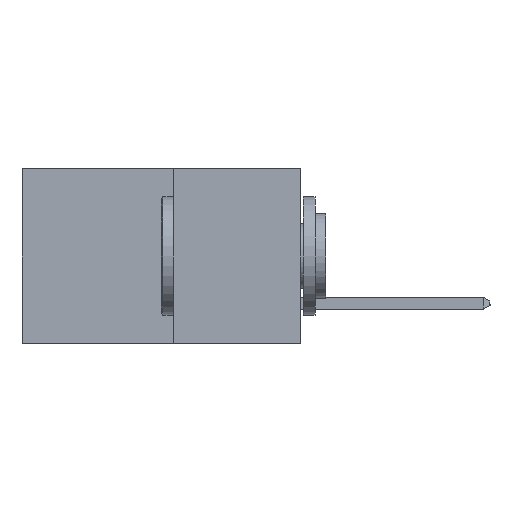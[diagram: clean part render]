
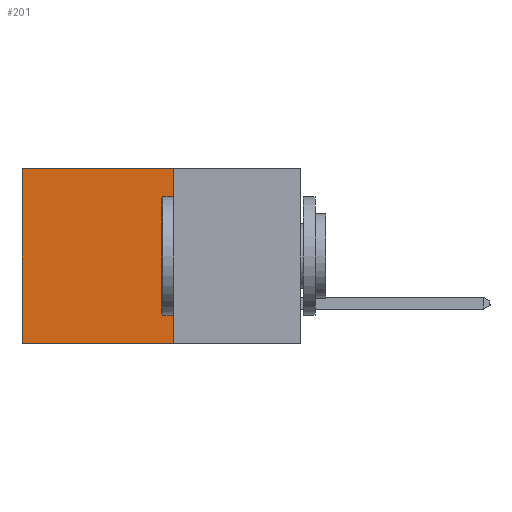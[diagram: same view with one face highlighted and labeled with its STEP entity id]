
A CAD part, left-side view. The second image highlights one B-rep face of the part: STEP entity #201.
In plain terms, the highlighted planar face has unit normal (-1, 0, 0).
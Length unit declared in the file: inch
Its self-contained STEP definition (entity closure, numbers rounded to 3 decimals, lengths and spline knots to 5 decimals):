
#201 = ADVANCED_FACE ( 'NONE', ( #12856 ), #9001, .F. ) ;
#291 = DIRECTION ( 'NONE',  ( 0., 1., 0. ) ) ;
#618 = ORIENTED_EDGE ( 'NONE', *, *, #7267, .T. ) ;
#1165 = ORIENTED_EDGE ( 'NONE', *, *, #3580, .F. ) ;
#1316 = LINE ( 'NONE', #10894, #13459 ) ;
#1512 = ORIENTED_EDGE ( 'NONE', *, *, #8063, .F. ) ;
#1718 = DIRECTION ( 'NONE',  ( 0., 0., -1. ) ) ;
#1719 = DIRECTION ( 'NONE',  ( 1., 0., 0. ) ) ;
#1788 = ORIENTED_EDGE ( 'NONE', *, *, #15020, .T. ) ;
#2161 = CARTESIAN_POINT ( 'NONE',  ( 0.277, 0.27, -0.37 ) ) ;
#2297 = CARTESIAN_POINT ( 'NONE',  ( 0.277, 0.59, 0. ) ) ;
#3491 = LINE ( 'NONE', #8458, #9470 ) ;
#3580 = EDGE_CURVE ( 'NONE', #7856, #14403, #13912, .T. ) ;
#3584 = CARTESIAN_POINT ( 'NONE',  ( 0.277, 0.59, -0.37 ) ) ;
#4010 = CARTESIAN_POINT ( 'NONE',  ( 0.277, 0.27, 0. ) ) ;
#4120 = VECTOR ( 'NONE', #291, 39.37008 ) ;
#6214 = DIRECTION ( 'NONE',  ( 0., 0., -1. ) ) ;
#7267 = EDGE_CURVE ( 'NONE', #9226, #14403, #3491, .T. ) ;
#7273 = LINE ( 'NONE', #4010, #4120 ) ;
#7856 = VERTEX_POINT ( 'NONE', #2161 ) ;
#8063 = EDGE_CURVE ( 'NONE', #14205, #7856, #1316, .T. ) ;
#8279 = VECTOR ( 'NONE', #10379, 39.37008 ) ;
#8379 = DIRECTION ( 'NONE',  ( 0., 0., -1. ) ) ;
#8458 = CARTESIAN_POINT ( 'NONE',  ( 0.277, 0.59, -0.37 ) ) ;
#9001 = PLANE ( 'NONE',  #9139 ) ;
#9139 = AXIS2_PLACEMENT_3D ( 'NONE', #11247, #1719, #1718 ) ;
#9226 = VERTEX_POINT ( 'NONE', #2297 ) ;
#9470 = VECTOR ( 'NONE', #8379, 39.37008 ) ;
#9526 = EDGE_LOOP ( 'NONE', ( #618, #1165, #1512, #1788 ) ) ;
#10379 = DIRECTION ( 'NONE',  ( 0., 1., 0. ) ) ;
#10894 = CARTESIAN_POINT ( 'NONE',  ( 0.277, 0.27, -0.37 ) ) ;
#11247 = CARTESIAN_POINT ( 'NONE',  ( 0.277, 0.27, -0.37 ) ) ;
#11522 = CARTESIAN_POINT ( 'NONE',  ( 0.277, 0.27, -0.37 ) ) ;
#12657 = CARTESIAN_POINT ( 'NONE',  ( 0.277, 0.27, 0. ) ) ;
#12856 = FACE_OUTER_BOUND ( 'NONE', #9526, .T. ) ;
#13459 = VECTOR ( 'NONE', #6214, 39.37008 ) ;
#13912 = LINE ( 'NONE', #11522, #8279 ) ;
#14205 = VERTEX_POINT ( 'NONE', #12657 ) ;
#14403 = VERTEX_POINT ( 'NONE', #3584 ) ;
#15020 = EDGE_CURVE ( 'NONE', #14205, #9226, #7273, .T. ) ;
